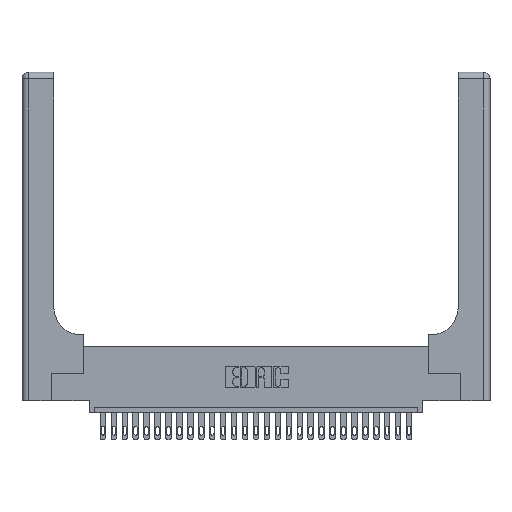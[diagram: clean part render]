
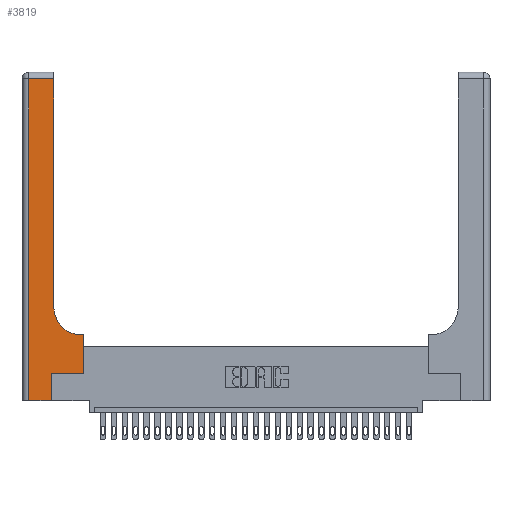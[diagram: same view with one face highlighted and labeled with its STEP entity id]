
A CAD part, top view. The second image highlights one B-rep face of the part: STEP entity #3819.
In plain terms, the highlighted planar face has unit normal (0, 0, 1).
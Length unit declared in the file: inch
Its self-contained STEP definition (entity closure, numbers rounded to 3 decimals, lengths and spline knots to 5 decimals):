
#97 = LINE ( 'NONE', #10255, #19227 ) ;
#822 = CARTESIAN_POINT ( 'NONE',  ( 0., 3., 0.37 ) ) ;
#1695 = CARTESIAN_POINT ( 'NONE',  ( 0.2915, 2.94, 0.37 ) ) ;
#1710 = DIRECTION ( 'NONE',  ( 0., -1., 0. ) ) ;
#2101 = ORIENTED_EDGE ( 'NONE', *, *, #17514, .T. ) ;
#2242 = CARTESIAN_POINT ( 'NONE',  ( 0.269, 0., 0.37 ) ) ;
#2244 = LINE ( 'NONE', #19536, #18520 ) ;
#3111 = ORIENTED_EDGE ( 'NONE', *, *, #5714, .T. ) ;
#3248 = CARTESIAN_POINT ( 'NONE',  ( 0.5415, 0.85, 0.37 ) ) ;
#3695 = DIRECTION ( 'NONE',  ( 1., 0., 0. ) ) ;
#3819 = ADVANCED_FACE ( 'NONE', ( #14098 ), #18595, .F. ) ;
#4180 = ORIENTED_EDGE ( 'NONE', *, *, #25265, .T. ) ;
#4798 = DIRECTION ( 'NONE',  ( 0., 1., 0. ) ) ;
#5714 = EDGE_CURVE ( 'NONE', #21758, #19069, #2244, .T. ) ;
#5922 = ORIENTED_EDGE ( 'NONE', *, *, #12405, .T. ) ;
#6668 = CARTESIAN_POINT ( 'NONE',  ( 0.06, 0., 0.37 ) ) ;
#7171 = ORIENTED_EDGE ( 'NONE', *, *, #26205, .T. ) ;
#7647 = EDGE_CURVE ( 'NONE', #9739, #27626, #9395, .T. ) ;
#8298 = ORIENTED_EDGE ( 'NONE', *, *, #21064, .T. ) ;
#8969 = VECTOR ( 'NONE', #19037, 39.37008 ) ;
#9097 = VERTEX_POINT ( 'NONE', #27888 ) ;
#9315 = ORIENTED_EDGE ( 'NONE', *, *, #26405, .T. ) ;
#9395 = LINE ( 'NONE', #15704, #14612 ) ;
#9606 = AXIS2_PLACEMENT_3D ( 'NONE', #3248, #16342, #22953 ) ;
#9739 = VERTEX_POINT ( 'NONE', #2242 ) ;
#9821 = CARTESIAN_POINT ( 'NONE',  ( 0.5585, 0.25, 0.37 ) ) ;
#10255 = CARTESIAN_POINT ( 'NONE',  ( 0., 0., 0.37 ) ) ;
#11630 = CARTESIAN_POINT ( 'NONE',  ( 0.06, 2.94, 0.37 ) ) ;
#11896 = LINE ( 'NONE', #24205, #26904 ) ;
#11972 = DIRECTION ( 'NONE',  ( 0., 0., -1. ) ) ;
#12405 = EDGE_CURVE ( 'NONE', #19069, #26490, #24958, .T. ) ;
#12866 = DIRECTION ( 'NONE',  ( 1., 0., 0. ) ) ;
#13425 = CARTESIAN_POINT ( 'NONE',  ( 0.2915, 3., 0.37 ) ) ;
#14098 = FACE_OUTER_BOUND ( 'NONE', #15500, .T. ) ;
#14612 = VECTOR ( 'NONE', #17928, 39.37008 ) ;
#14637 = VECTOR ( 'NONE', #18192, 39.37008 ) ;
#14871 = LINE ( 'NONE', #18941, #8969 ) ;
#15500 = EDGE_LOOP ( 'NONE', ( #9315, #3111, #5922, #7171, #27141, #8298, #2101, #21920, #4180 ) ) ;
#15704 = CARTESIAN_POINT ( 'NONE',  ( 0.269, 0., 0.37 ) ) ;
#16342 = DIRECTION ( 'NONE',  ( 0., 0., -1. ) ) ;
#16345 = VERTEX_POINT ( 'NONE', #9821 ) ;
#17102 = LINE ( 'NONE', #18494, #14637 ) ;
#17514 = EDGE_CURVE ( 'NONE', #16345, #28648, #14871, .T. ) ;
#17533 = CARTESIAN_POINT ( 'NONE',  ( 0.2915, 0.85, 0.37 ) ) ;
#17928 = DIRECTION ( 'NONE',  ( 0., 1., 0. ) ) ;
#18192 = DIRECTION ( 'NONE',  ( -1., 0., 0. ) ) ;
#18494 = CARTESIAN_POINT ( 'NONE',  ( 0.2915, 0.6, 0.37 ) ) ;
#18520 = VECTOR ( 'NONE', #27641, 39.37008 ) ;
#18595 = PLANE ( 'NONE',  #19749 ) ;
#18721 = VERTEX_POINT ( 'NONE', #17533 ) ;
#18941 = CARTESIAN_POINT ( 'NONE',  ( 0.5585, 0.25, 0.37 ) ) ;
#19037 = DIRECTION ( 'NONE',  ( 0., 1., 0. ) ) ;
#19069 = VERTEX_POINT ( 'NONE', #11630 ) ;
#19183 = CARTESIAN_POINT ( 'NONE',  ( 0.06, 3., 0.37 ) ) ;
#19227 = VECTOR ( 'NONE', #3695, 39.37008 ) ;
#19536 = CARTESIAN_POINT ( 'NONE',  ( 0., 2.94, 0.37 ) ) ;
#19749 = AXIS2_PLACEMENT_3D ( 'NONE', #822, #11972, #20833 ) ;
#19892 = LINE ( 'NONE', #13425, #27208 ) ;
#20833 = DIRECTION ( 'NONE',  ( -1., 0., 0. ) ) ;
#21064 = EDGE_CURVE ( 'NONE', #27626, #16345, #11896, .T. ) ;
#21758 = VERTEX_POINT ( 'NONE', #1695 ) ;
#21920 = ORIENTED_EDGE ( 'NONE', *, *, #26557, .T. ) ;
#22953 = DIRECTION ( 'NONE',  ( 1., 0., 0. ) ) ;
#24205 = CARTESIAN_POINT ( 'NONE',  ( 0.269, 0.25, 0.37 ) ) ;
#24958 = LINE ( 'NONE', #19183, #27405 ) ;
#25265 = EDGE_CURVE ( 'NONE', #9097, #18721, #26585, .T. ) ;
#26205 = EDGE_CURVE ( 'NONE', #26490, #9739, #97, .T. ) ;
#26405 = EDGE_CURVE ( 'NONE', #18721, #21758, #19892, .T. ) ;
#26490 = VERTEX_POINT ( 'NONE', #6668 ) ;
#26557 = EDGE_CURVE ( 'NONE', #28648, #9097, #17102, .T. ) ;
#26585 = CIRCLE ( 'NONE', #9606, 0.25 ) ;
#26742 = CARTESIAN_POINT ( 'NONE',  ( 0.269, 0.25, 0.37 ) ) ;
#26904 = VECTOR ( 'NONE', #12866, 39.37008 ) ;
#27141 = ORIENTED_EDGE ( 'NONE', *, *, #7647, .T. ) ;
#27208 = VECTOR ( 'NONE', #4798, 39.37008 ) ;
#27405 = VECTOR ( 'NONE', #1710, 39.37008 ) ;
#27626 = VERTEX_POINT ( 'NONE', #26742 ) ;
#27641 = DIRECTION ( 'NONE',  ( -1., 0., 0. ) ) ;
#27888 = CARTESIAN_POINT ( 'NONE',  ( 0.5415, 0.6, 0.37 ) ) ;
#28648 = VERTEX_POINT ( 'NONE', #28763 ) ;
#28763 = CARTESIAN_POINT ( 'NONE',  ( 0.5585, 0.6, 0.37 ) ) ;
